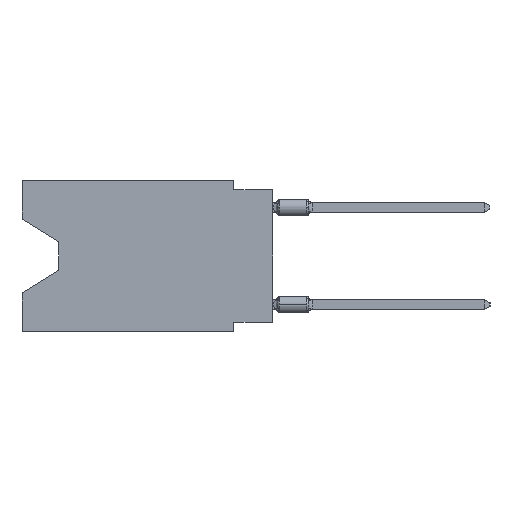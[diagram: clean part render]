
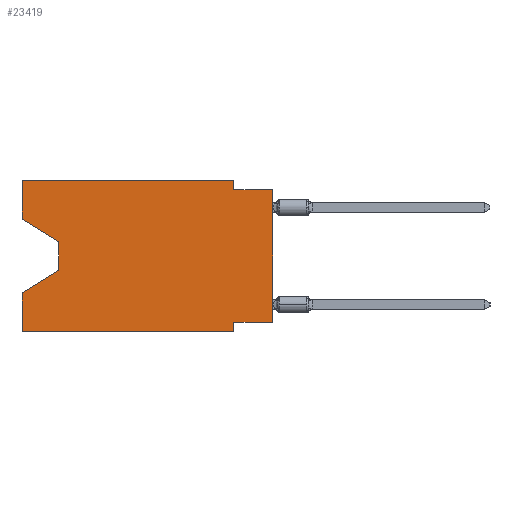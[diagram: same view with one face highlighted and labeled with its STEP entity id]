
A CAD part, left-side view. The second image highlights one B-rep face of the part: STEP entity #23419.
In plain terms, the highlighted planar face has unit normal (-1, 0, 0).
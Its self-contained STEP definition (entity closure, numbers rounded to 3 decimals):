
#165 = VECTOR ( 'NONE', #1990, 1000. ) ;
#193 = VECTOR ( 'NONE', #32544, 1000. ) ;
#634 = ORIENTED_EDGE ( 'NONE', *, *, #27108, .T. ) ;
#1880 = DIRECTION ( 'NONE',  ( 0., 1., 0. ) ) ;
#1990 = DIRECTION ( 'NONE',  ( 0., 0., -1. ) ) ;
#2233 = ORIENTED_EDGE ( 'NONE', *, *, #22246, .F. ) ;
#2949 = VERTEX_POINT ( 'NONE', #5524 ) ;
#3579 = VECTOR ( 'NONE', #28430, 1000. ) ;
#3940 = VERTEX_POINT ( 'NONE', #30237 ) ;
#4665 = ORIENTED_EDGE ( 'NONE', *, *, #34422, .T. ) ;
#4688 = LINE ( 'NONE', #20313, #25211 ) ;
#4859 = FACE_OUTER_BOUND ( 'NONE', #15281, .T. ) ;
#5244 = DIRECTION ( 'NONE',  ( 0., 0.855, -0.519 ) ) ;
#5255 = CARTESIAN_POINT ( 'NONE',  ( 0., 13.97, -5.893 ) ) ;
#5446 = CARTESIAN_POINT ( 'NONE',  ( 0., 13.97, -5.893 ) ) ;
#5524 = CARTESIAN_POINT ( 'NONE',  ( 0., 13.97, -4.013 ) ) ;
#5679 = VERTEX_POINT ( 'NONE', #22318 ) ;
#6091 = DIRECTION ( 'NONE',  ( 0., 0., -1. ) ) ;
#6599 = VERTEX_POINT ( 'NONE', #23402 ) ;
#6966 = VERTEX_POINT ( 'NONE', #26553 ) ;
#8084 = LINE ( 'NONE', #20315, #37611 ) ;
#8099 = ORIENTED_EDGE ( 'NONE', *, *, #34923, .F. ) ;
#8485 = LINE ( 'NONE', #17296, #10348 ) ;
#8689 = DIRECTION ( 'NONE',  ( 0., -0.855, -0.519 ) ) ;
#8732 = ORIENTED_EDGE ( 'NONE', *, *, #20485, .F. ) ;
#9298 = EDGE_CURVE ( 'NONE', #6966, #25546, #26433, .T. ) ;
#9746 = DIRECTION ( 'NONE',  ( 0., -1., 0. ) ) ;
#10299 = CARTESIAN_POINT ( 'NONE',  ( 0., 16.383, -9.906 ) ) ;
#10348 = VECTOR ( 'NONE', #17692, 1000. ) ;
#10435 = ORIENTED_EDGE ( 'NONE', *, *, #39282, .T. ) ;
#10852 = PLANE ( 'NONE',  #29668 ) ;
#11061 = ORIENTED_EDGE ( 'NONE', *, *, #25360, .F. ) ;
#11415 = ORIENTED_EDGE ( 'NONE', *, *, #25485, .T. ) ;
#12427 = CARTESIAN_POINT ( 'NONE',  ( 0., 0., -9.271 ) ) ;
#12529 = VERTEX_POINT ( 'NONE', #27305 ) ;
#12745 = LINE ( 'NONE', #24969, #21322 ) ;
#13655 = ORIENTED_EDGE ( 'NONE', *, *, #32993, .F. ) ;
#14610 = ORIENTED_EDGE ( 'NONE', *, *, #9298, .F. ) ;
#15281 = EDGE_LOOP ( 'NONE', ( #634, #4665, #35323, #15331, #10435, #11061, #8732, #11415, #2233, #14610, #13655, #8099 ) ) ;
#15331 = ORIENTED_EDGE ( 'NONE', *, *, #23388, .F. ) ;
#15877 = VERTEX_POINT ( 'NONE', #12427 ) ;
#17296 = CARTESIAN_POINT ( 'NONE',  ( 0., 16.383, 0. ) ) ;
#17692 = DIRECTION ( 'NONE',  ( 0., -1., 0. ) ) ;
#18904 = LINE ( 'NONE', #30710, #32225 ) ;
#19278 = VECTOR ( 'NONE', #8689, 1000. ) ;
#20313 = CARTESIAN_POINT ( 'NONE',  ( 0., 16.383, 0. ) ) ;
#20315 = CARTESIAN_POINT ( 'NONE',  ( 0., 0., -9.271 ) ) ;
#20347 = LINE ( 'NONE', #23745, #193 ) ;
#20485 = EDGE_CURVE ( 'NONE', #15877, #22199, #8084, .T. ) ;
#20675 = DIRECTION ( 'NONE',  ( 1., 0., 0. ) ) ;
#21322 = VECTOR ( 'NONE', #9746, 1000. ) ;
#21400 = VERTEX_POINT ( 'NONE', #5255 ) ;
#22110 = LINE ( 'NONE', #37539, #28405 ) ;
#22199 = VERTEX_POINT ( 'NONE', #26150 ) ;
#22246 = EDGE_CURVE ( 'NONE', #25546, #27149, #20347, .T. ) ;
#22318 = CARTESIAN_POINT ( 'NONE',  ( 0., 16.383, -2.546 ) ) ;
#22722 = DIRECTION ( 'NONE',  ( 0., 0., 1. ) ) ;
#22759 = VECTOR ( 'NONE', #25421, 1000. ) ;
#22996 = CARTESIAN_POINT ( 'NONE',  ( 0., 2.54, -0.635 ) ) ;
#23077 = DIRECTION ( 'NONE',  ( 0., 0., -1. ) ) ;
#23120 = CARTESIAN_POINT ( 'NONE',  ( 0., 16.383, -2.546 ) ) ;
#23388 = EDGE_CURVE ( 'NONE', #34917, #6599, #22110, .T. ) ;
#23402 = CARTESIAN_POINT ( 'NONE',  ( 0., 16.383, -7.36 ) ) ;
#23419 = ADVANCED_FACE ( 'NONE', ( #4859 ), #10852, .F. ) ;
#23482 = LINE ( 'NONE', #5446, #39091 ) ;
#23745 = CARTESIAN_POINT ( 'NONE',  ( 0., 0., -0.635 ) ) ;
#24969 = CARTESIAN_POINT ( 'NONE',  ( 0., 16.383, -9.906 ) ) ;
#25211 = VECTOR ( 'NONE', #22722, 1000. ) ;
#25360 = EDGE_CURVE ( 'NONE', #22199, #12529, #34615, .T. ) ;
#25421 = DIRECTION ( 'NONE',  ( 0., 0., -1. ) ) ;
#25485 = EDGE_CURVE ( 'NONE', #15877, #27149, #31413, .T. ) ;
#25546 = VERTEX_POINT ( 'NONE', #22996 ) ;
#26150 = CARTESIAN_POINT ( 'NONE',  ( 0., 2.54, -9.271 ) ) ;
#26433 = LINE ( 'NONE', #28657, #165 ) ;
#26553 = CARTESIAN_POINT ( 'NONE',  ( 0., 2.54, 0. ) ) ;
#27108 = EDGE_CURVE ( 'NONE', #5679, #2949, #32329, .T. ) ;
#27149 = VERTEX_POINT ( 'NONE', #35338 ) ;
#27305 = CARTESIAN_POINT ( 'NONE',  ( 0., 2.54, -9.906 ) ) ;
#27541 = EDGE_CURVE ( 'NONE', #21400, #6599, #23482, .T. ) ;
#28405 = VECTOR ( 'NONE', #34314, 1000. ) ;
#28430 = DIRECTION ( 'NONE',  ( 0., 0., 1. ) ) ;
#28657 = CARTESIAN_POINT ( 'NONE',  ( 0., 2.54, 0. ) ) ;
#29668 = AXIS2_PLACEMENT_3D ( 'NONE', #35498, #20675, #23077 ) ;
#30237 = CARTESIAN_POINT ( 'NONE',  ( 0., 16.383, 0. ) ) ;
#30710 = CARTESIAN_POINT ( 'NONE',  ( 0., 13.97, -4.013 ) ) ;
#31413 = LINE ( 'NONE', #37647, #3579 ) ;
#32225 = VECTOR ( 'NONE', #6091, 1000. ) ;
#32329 = LINE ( 'NONE', #23120, #19278 ) ;
#32544 = DIRECTION ( 'NONE',  ( 0., -1., 0. ) ) ;
#32993 = EDGE_CURVE ( 'NONE', #3940, #6966, #8485, .T. ) ;
#34314 = DIRECTION ( 'NONE',  ( 0., 0., 1. ) ) ;
#34422 = EDGE_CURVE ( 'NONE', #2949, #21400, #18904, .T. ) ;
#34615 = LINE ( 'NONE', #37831, #22759 ) ;
#34917 = VERTEX_POINT ( 'NONE', #10299 ) ;
#34923 = EDGE_CURVE ( 'NONE', #5679, #3940, #4688, .T. ) ;
#35323 = ORIENTED_EDGE ( 'NONE', *, *, #27541, .T. ) ;
#35338 = CARTESIAN_POINT ( 'NONE',  ( 0., 0., -0.635 ) ) ;
#35498 = CARTESIAN_POINT ( 'NONE',  ( 0., 16.383, 0. ) ) ;
#37539 = CARTESIAN_POINT ( 'NONE',  ( 0., 16.383, 0. ) ) ;
#37611 = VECTOR ( 'NONE', #1880, 1000. ) ;
#37647 = CARTESIAN_POINT ( 'NONE',  ( 0., 0., 0. ) ) ;
#37831 = CARTESIAN_POINT ( 'NONE',  ( 0., 2.54, -9.906 ) ) ;
#39091 = VECTOR ( 'NONE', #5244, 1000. ) ;
#39282 = EDGE_CURVE ( 'NONE', #34917, #12529, #12745, .T. ) ;
